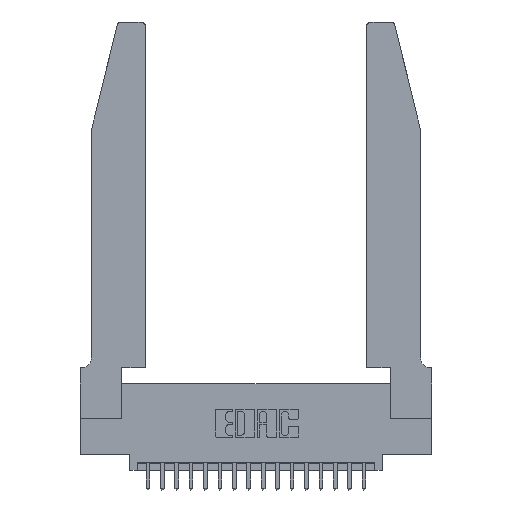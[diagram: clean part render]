
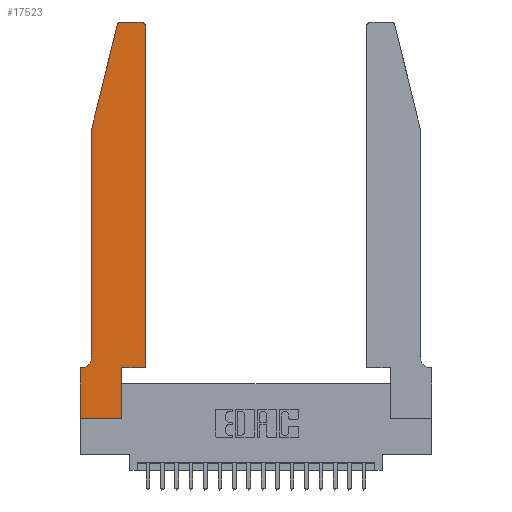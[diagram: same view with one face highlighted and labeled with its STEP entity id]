
A CAD part, top view. The second image highlights one B-rep face of the part: STEP entity #17523.
In plain terms, the highlighted planar face has unit normal (0, 0, 1).
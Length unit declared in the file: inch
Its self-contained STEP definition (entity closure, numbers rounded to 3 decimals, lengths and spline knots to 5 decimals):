
#50 = EDGE_CURVE ( 'NONE', #6561, #12949, #13495, .T. ) ;
#210 = DIRECTION ( 'NONE',  ( 0., 1., 0. ) ) ;
#257 = EDGE_CURVE ( 'NONE', #16593, #8250, #14994, .T. ) ;
#698 = EDGE_CURVE ( 'NONE', #8433, #6561, #11961, .T. ) ;
#804 = CARTESIAN_POINT ( 'NONE',  ( 0., 0.35, 0.37 ) ) ;
#906 = DIRECTION ( 'NONE',  ( 1., 0., 0. ) ) ;
#1248 = VERTEX_POINT ( 'NONE', #13871 ) ;
#1556 = LINE ( 'NONE', #2801, #13160 ) ;
#1650 = CARTESIAN_POINT ( 'NONE',  ( 0., 0., 0.37 ) ) ;
#1708 = DIRECTION ( 'NONE',  ( -1., 0., 0. ) ) ;
#2106 = VERTEX_POINT ( 'NONE', #1650 ) ;
#2122 = DIRECTION ( 'NONE',  ( 0., 0., 1. ) ) ;
#2801 = CARTESIAN_POINT ( 'NONE',  ( 0., 0., 0.37 ) ) ;
#2891 = EDGE_CURVE ( 'NONE', #18404, #12130, #13781, .T. ) ;
#3198 = CARTESIAN_POINT ( 'NONE',  ( 0.284, 2.75, 0.37 ) ) ;
#3216 = ORIENTED_EDGE ( 'NONE', *, *, #9591, .T. ) ;
#3517 = CARTESIAN_POINT ( 'NONE',  ( 0.4205, 2.72, 0.37 ) ) ;
#3552 = AXIS2_PLACEMENT_3D ( 'NONE', #3517, #16179, #18049 ) ;
#3903 = CIRCLE ( 'NONE', #15133, 0.03 ) ;
#4496 = DIRECTION ( 'NONE',  ( 0., 1., 0. ) ) ;
#5476 = ORIENTED_EDGE ( 'NONE', *, *, #698, .T. ) ;
#5626 = DIRECTION ( 'NONE',  ( 0., 0., -1. ) ) ;
#6194 = DIRECTION ( 'NONE',  ( 0., 0., 1. ) ) ;
#6276 = CARTESIAN_POINT ( 'NONE',  ( 0.25487, 2.72718, 0.37 ) ) ;
#6387 = DIRECTION ( 'NONE',  ( 1., 0., 0. ) ) ;
#6561 = VERTEX_POINT ( 'NONE', #15970 ) ;
#6826 = EDGE_CURVE ( 'NONE', #1248, #17283, #9379, .T. ) ;
#6978 = VECTOR ( 'NONE', #18555, 39.37008 ) ;
#7021 = CARTESIAN_POINT ( 'NONE',  ( 0.0755, 0.35, 0.37 ) ) ;
#7036 = CARTESIAN_POINT ( 'NONE',  ( 0., 0.35, 0.37 ) ) ;
#7400 = VECTOR ( 'NONE', #4496, 39.37008 ) ;
#7429 = CARTESIAN_POINT ( 'NONE',  ( 0.0755, 2., 0.37 ) ) ;
#7451 = AXIS2_PLACEMENT_3D ( 'NONE', #15244, #5626, #10550 ) ;
#8082 = LINE ( 'NONE', #19530, #19432 ) ;
#8250 = VERTEX_POINT ( 'NONE', #18343 ) ;
#8433 = VERTEX_POINT ( 'NONE', #20900 ) ;
#8560 = DIRECTION ( 'NONE',  ( 1., 0., 0. ) ) ;
#8595 = ORIENTED_EDGE ( 'NONE', *, *, #257, .T. ) ;
#8608 = CARTESIAN_POINT ( 'NONE',  ( 0.2865, 0.35, 0.37 ) ) ;
#8878 = CARTESIAN_POINT ( 'NONE',  ( 0.4505, 0.35, 0.37 ) ) ;
#8978 = VECTOR ( 'NONE', #11656, 39.37008 ) ;
#9074 = CARTESIAN_POINT ( 'NONE',  ( 0.4505, 0.35, 0.37 ) ) ;
#9379 = CIRCLE ( 'NONE', #3552, 0.03 ) ;
#9591 = EDGE_CURVE ( 'NONE', #12130, #12586, #19223, .T. ) ;
#9609 = VECTOR ( 'NONE', #906, 39.37008 ) ;
#10023 = VECTOR ( 'NONE', #18777, 39.37008 ) ;
#10066 = ORIENTED_EDGE ( 'NONE', *, *, #20914, .T. ) ;
#10116 = VECTOR ( 'NONE', #16416, 39.37008 ) ;
#10550 = DIRECTION ( 'NONE',  ( -1., 0., 0. ) ) ;
#10947 = ORIENTED_EDGE ( 'NONE', *, *, #17186, .T. ) ;
#11403 = ORIENTED_EDGE ( 'NONE', *, *, #50, .T. ) ;
#11587 = CARTESIAN_POINT ( 'NONE',  ( 0.0755, 2., 0.37 ) ) ;
#11656 = DIRECTION ( 'NONE',  ( -0.239, -0.971, 0. ) ) ;
#11961 = CIRCLE ( 'NONE', #7451, 0.07 ) ;
#12098 = ORIENTED_EDGE ( 'NONE', *, *, #14421, .T. ) ;
#12130 = VERTEX_POINT ( 'NONE', #8608 ) ;
#12427 = ORIENTED_EDGE ( 'NONE', *, *, #17073, .T. ) ;
#12586 = VERTEX_POINT ( 'NONE', #17572 ) ;
#12621 = ORIENTED_EDGE ( 'NONE', *, *, #19959, .T. ) ;
#12644 = CARTESIAN_POINT ( 'NONE',  ( 0.4205, 2.75, 0.37 ) ) ;
#12709 = CARTESIAN_POINT ( 'NONE',  ( 0.284, 2.72, 0.37 ) ) ;
#12949 = VERTEX_POINT ( 'NONE', #804 ) ;
#13160 = VECTOR ( 'NONE', #6387, 39.37008 ) ;
#13495 = LINE ( 'NONE', #7021, #6978 ) ;
#13781 = LINE ( 'NONE', #19683, #18856 ) ;
#13871 = CARTESIAN_POINT ( 'NONE',  ( 0.4505, 2.72, 0.37 ) ) ;
#14074 = CARTESIAN_POINT ( 'NONE',  ( 0.2865, 0., 0.37 ) ) ;
#14235 = EDGE_CURVE ( 'NONE', #19061, #16593, #3903, .T. ) ;
#14409 = LINE ( 'NONE', #9074, #7400 ) ;
#14421 = EDGE_CURVE ( 'NONE', #12949, #2106, #16388, .T. ) ;
#14994 = LINE ( 'NONE', #11587, #8978 ) ;
#15133 = AXIS2_PLACEMENT_3D ( 'NONE', #12709, #6194, #15932 ) ;
#15244 = CARTESIAN_POINT ( 'NONE',  ( 0.0055, 0.42, 0.37 ) ) ;
#15671 = FACE_OUTER_BOUND ( 'NONE', #18695, .T. ) ;
#15932 = DIRECTION ( 'NONE',  ( 1., 0., 0. ) ) ;
#15970 = CARTESIAN_POINT ( 'NONE',  ( 0.0055, 0.35, 0.37 ) ) ;
#16179 = DIRECTION ( 'NONE',  ( 0., 0., 1. ) ) ;
#16388 = LINE ( 'NONE', #19856, #10116 ) ;
#16398 = AXIS2_PLACEMENT_3D ( 'NONE', #7036, #2122, #8560 ) ;
#16416 = DIRECTION ( 'NONE',  ( 0., -1., 0. ) ) ;
#16593 = VERTEX_POINT ( 'NONE', #6276 ) ;
#17073 = EDGE_CURVE ( 'NONE', #12586, #1248, #14409, .T. ) ;
#17186 = EDGE_CURVE ( 'NONE', #2106, #18404, #1556, .T. ) ;
#17283 = VERTEX_POINT ( 'NONE', #12644 ) ;
#17523 = ADVANCED_FACE ( 'NONE', ( #15671 ), #19791, .T. ) ;
#17572 = CARTESIAN_POINT ( 'NONE',  ( 0.4505, 0.35, 0.37 ) ) ;
#18049 = DIRECTION ( 'NONE',  ( 1., 0., 0. ) ) ;
#18208 = ORIENTED_EDGE ( 'NONE', *, *, #6826, .T. ) ;
#18343 = CARTESIAN_POINT ( 'NONE',  ( 0.0755, 2., 0.37 ) ) ;
#18404 = VERTEX_POINT ( 'NONE', #14074 ) ;
#18555 = DIRECTION ( 'NONE',  ( -1., 0., 0. ) ) ;
#18695 = EDGE_LOOP ( 'NONE', ( #12621, #19905, #8595, #10066, #5476, #11403, #12098, #10947, #20627, #3216, #12427, #18208 ) ) ;
#18777 = DIRECTION ( 'NONE',  ( 0., -1., 0. ) ) ;
#18856 = VECTOR ( 'NONE', #210, 39.37008 ) ;
#19061 = VERTEX_POINT ( 'NONE', #3198 ) ;
#19223 = LINE ( 'NONE', #8878, #9609 ) ;
#19432 = VECTOR ( 'NONE', #1708, 39.37008 ) ;
#19530 = CARTESIAN_POINT ( 'NONE',  ( 0.2605, 2.75, 0.37 ) ) ;
#19683 = CARTESIAN_POINT ( 'NONE',  ( 0.2865, 0.35, 0.37 ) ) ;
#19791 = PLANE ( 'NONE',  #16398 ) ;
#19856 = CARTESIAN_POINT ( 'NONE',  ( 0., 0., 0.37 ) ) ;
#19905 = ORIENTED_EDGE ( 'NONE', *, *, #14235, .T. ) ;
#19959 = EDGE_CURVE ( 'NONE', #17283, #19061, #8082, .T. ) ;
#20143 = LINE ( 'NONE', #7429, #10023 ) ;
#20627 = ORIENTED_EDGE ( 'NONE', *, *, #2891, .T. ) ;
#20900 = CARTESIAN_POINT ( 'NONE',  ( 0.0755, 0.42, 0.37 ) ) ;
#20914 = EDGE_CURVE ( 'NONE', #8250, #8433, #20143, .T. ) ;
